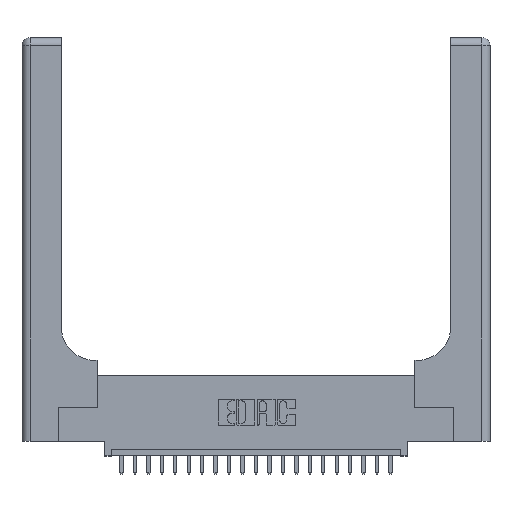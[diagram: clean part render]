
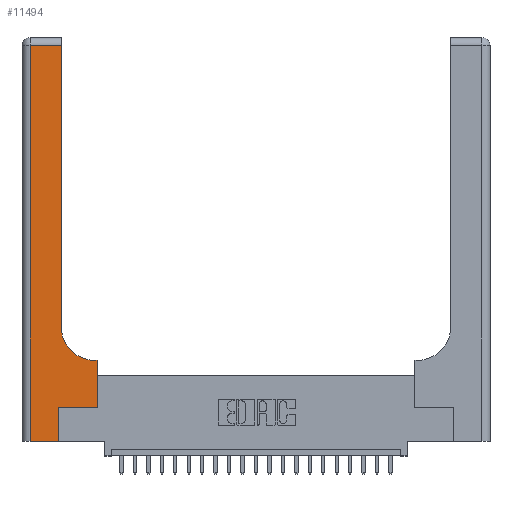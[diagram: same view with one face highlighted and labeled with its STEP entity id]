
A CAD part, top view. The second image highlights one B-rep face of the part: STEP entity #11494.
In plain terms, the highlighted planar face has unit normal (0, 0, 1).
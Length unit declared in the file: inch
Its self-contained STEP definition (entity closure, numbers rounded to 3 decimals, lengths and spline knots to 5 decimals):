
#153 = ORIENTED_EDGE ( 'NONE', *, *, #8964, .T. ) ;
#203 = AXIS2_PLACEMENT_3D ( 'NONE', #23292, #6483, #3095 ) ;
#204 = EDGE_CURVE ( 'NONE', #9136, #23179, #3851, .T. ) ;
#211 = PLANE ( 'NONE',  #7662 ) ;
#289 = LINE ( 'NONE', #3054, #4065 ) ;
#326 = CARTESIAN_POINT ( 'NONE',  ( 0.06, 0., 0.37 ) ) ;
#746 = CARTESIAN_POINT ( 'NONE',  ( 0.5585, 0.25, 0.37 ) ) ;
#1947 = CARTESIAN_POINT ( 'NONE',  ( 0.269, 0., 0.37 ) ) ;
#2049 = LINE ( 'NONE', #14517, #4045 ) ;
#2868 = CARTESIAN_POINT ( 'NONE',  ( 0.5415, 0.6, 0.37 ) ) ;
#3054 = CARTESIAN_POINT ( 'NONE',  ( 0.5585, 0.25, 0.37 ) ) ;
#3095 = DIRECTION ( 'NONE',  ( 1., 0., 0. ) ) ;
#3851 = LINE ( 'NONE', #10374, #9031 ) ;
#4045 = VECTOR ( 'NONE', #10992, 39.37008 ) ;
#4065 = VECTOR ( 'NONE', #17806, 39.37008 ) ;
#4075 = LINE ( 'NONE', #10470, #23160 ) ;
#4114 = VECTOR ( 'NONE', #14689, 39.37008 ) ;
#5146 = VERTEX_POINT ( 'NONE', #10585 ) ;
#6033 = DIRECTION ( 'NONE',  ( -1., 0., 0. ) ) ;
#6483 = DIRECTION ( 'NONE',  ( 0., 0., -1. ) ) ;
#6546 = CARTESIAN_POINT ( 'NONE',  ( 0., 2.94, 0.37 ) ) ;
#6763 = CARTESIAN_POINT ( 'NONE',  ( 0.2915, 3., 0.37 ) ) ;
#6778 = VECTOR ( 'NONE', #22246, 39.37008 ) ;
#6904 = EDGE_CURVE ( 'NONE', #12407, #9136, #8528, .T. ) ;
#7382 = CARTESIAN_POINT ( 'NONE',  ( 0.06, 3., 0.37 ) ) ;
#7410 = CARTESIAN_POINT ( 'NONE',  ( 0.06, 2.94, 0.37 ) ) ;
#7662 = AXIS2_PLACEMENT_3D ( 'NONE', #22627, #18963, #6033 ) ;
#7690 = ORIENTED_EDGE ( 'NONE', *, *, #13740, .T. ) ;
#8528 = LINE ( 'NONE', #7382, #6778 ) ;
#8651 = VERTEX_POINT ( 'NONE', #18022 ) ;
#8964 = EDGE_CURVE ( 'NONE', #8651, #12407, #16679, .T. ) ;
#9031 = VECTOR ( 'NONE', #21273, 39.37008 ) ;
#9136 = VERTEX_POINT ( 'NONE', #326 ) ;
#9430 = ORIENTED_EDGE ( 'NONE', *, *, #16124, .T. ) ;
#10256 = DIRECTION ( 'NONE',  ( -1., 0., 0. ) ) ;
#10374 = CARTESIAN_POINT ( 'NONE',  ( 0., 0., 0.37 ) ) ;
#10470 = CARTESIAN_POINT ( 'NONE',  ( 0.269, 0.25, 0.37 ) ) ;
#10495 = DIRECTION ( 'NONE',  ( 0., 1., 0. ) ) ;
#10585 = CARTESIAN_POINT ( 'NONE',  ( 0.269, 0.25, 0.37 ) ) ;
#10992 = DIRECTION ( 'NONE',  ( -1., 0., 0. ) ) ;
#11494 = ADVANCED_FACE ( 'NONE', ( #15371 ), #211, .F. ) ;
#11982 = ORIENTED_EDGE ( 'NONE', *, *, #17020, .T. ) ;
#12407 = VERTEX_POINT ( 'NONE', #7410 ) ;
#12492 = ORIENTED_EDGE ( 'NONE', *, *, #22746, .T. ) ;
#12832 = ORIENTED_EDGE ( 'NONE', *, *, #14690, .T. ) ;
#13004 = VERTEX_POINT ( 'NONE', #21710 ) ;
#13196 = VERTEX_POINT ( 'NONE', #19042 ) ;
#13432 = EDGE_CURVE ( 'NONE', #13196, #18985, #2049, .T. ) ;
#13740 = EDGE_CURVE ( 'NONE', #5146, #17307, #4075, .T. ) ;
#13907 = LINE ( 'NONE', #1947, #4114 ) ;
#14517 = CARTESIAN_POINT ( 'NONE',  ( 0.2915, 0.6, 0.37 ) ) ;
#14689 = DIRECTION ( 'NONE',  ( 0., 1., 0. ) ) ;
#14690 = EDGE_CURVE ( 'NONE', #13004, #8651, #16711, .T. ) ;
#14912 = VECTOR ( 'NONE', #10256, 39.37008 ) ;
#15371 = FACE_OUTER_BOUND ( 'NONE', #21700, .T. ) ;
#16124 = EDGE_CURVE ( 'NONE', #23179, #5146, #13907, .T. ) ;
#16591 = ORIENTED_EDGE ( 'NONE', *, *, #13432, .T. ) ;
#16609 = CIRCLE ( 'NONE', #203, 0.25 ) ;
#16679 = LINE ( 'NONE', #6546, #14912 ) ;
#16711 = LINE ( 'NONE', #6763, #23988 ) ;
#16844 = ORIENTED_EDGE ( 'NONE', *, *, #204, .T. ) ;
#17020 = EDGE_CURVE ( 'NONE', #17307, #13196, #289, .T. ) ;
#17307 = VERTEX_POINT ( 'NONE', #746 ) ;
#17719 = DIRECTION ( 'NONE',  ( 1., 0., 0. ) ) ;
#17806 = DIRECTION ( 'NONE',  ( 0., 1., 0. ) ) ;
#18022 = CARTESIAN_POINT ( 'NONE',  ( 0.2915, 2.94, 0.37 ) ) ;
#18321 = ORIENTED_EDGE ( 'NONE', *, *, #6904, .T. ) ;
#18737 = CARTESIAN_POINT ( 'NONE',  ( 0.269, 0., 0.37 ) ) ;
#18963 = DIRECTION ( 'NONE',  ( 0., 0., -1. ) ) ;
#18985 = VERTEX_POINT ( 'NONE', #2868 ) ;
#19042 = CARTESIAN_POINT ( 'NONE',  ( 0.5585, 0.6, 0.37 ) ) ;
#21273 = DIRECTION ( 'NONE',  ( 1., 0., 0. ) ) ;
#21700 = EDGE_LOOP ( 'NONE', ( #12832, #153, #18321, #16844, #9430, #7690, #11982, #16591, #12492 ) ) ;
#21710 = CARTESIAN_POINT ( 'NONE',  ( 0.2915, 0.85, 0.37 ) ) ;
#22246 = DIRECTION ( 'NONE',  ( 0., -1., 0. ) ) ;
#22627 = CARTESIAN_POINT ( 'NONE',  ( 0., 3., 0.37 ) ) ;
#22746 = EDGE_CURVE ( 'NONE', #18985, #13004, #16609, .T. ) ;
#23160 = VECTOR ( 'NONE', #17719, 39.37008 ) ;
#23179 = VERTEX_POINT ( 'NONE', #18737 ) ;
#23292 = CARTESIAN_POINT ( 'NONE',  ( 0.5415, 0.85, 0.37 ) ) ;
#23988 = VECTOR ( 'NONE', #10495, 39.37008 ) ;
